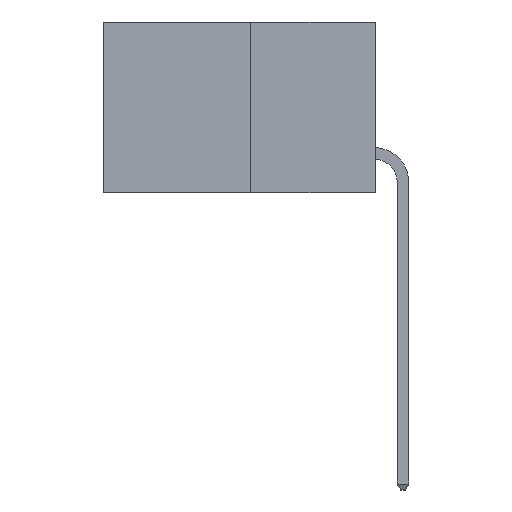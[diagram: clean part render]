
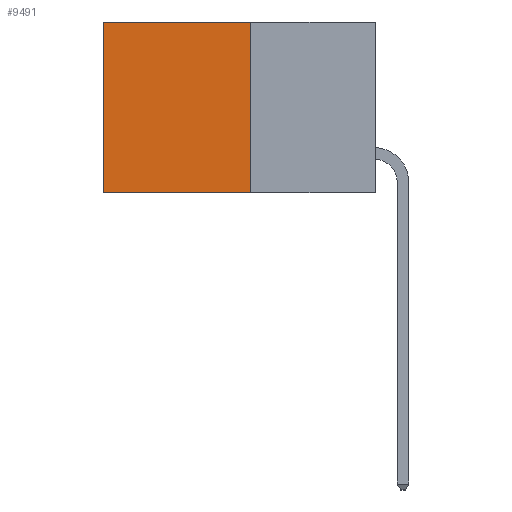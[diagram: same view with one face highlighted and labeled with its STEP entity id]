
A CAD part, left-side view. The second image highlights one B-rep face of the part: STEP entity #9491.
In plain terms, the highlighted planar face has unit normal (-1, 0, 0).
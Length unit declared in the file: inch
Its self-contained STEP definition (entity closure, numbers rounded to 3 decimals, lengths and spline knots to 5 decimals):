
#1117 = VECTOR ( 'NONE', #10026, 39.37008 ) ;
#1329 = VERTEX_POINT ( 'NONE', #5343 ) ;
#1611 = EDGE_CURVE ( 'NONE', #6706, #4238, #9862, .T. ) ;
#2186 = ORIENTED_EDGE ( 'NONE', *, *, #1611, .T. ) ;
#2219 = CARTESIAN_POINT ( 'NONE',  ( 0.277, 0.27, -0.37 ) ) ;
#2989 = VECTOR ( 'NONE', #11849, 39.37008 ) ;
#3197 = VERTEX_POINT ( 'NONE', #16836 ) ;
#3988 = EDGE_LOOP ( 'NONE', ( #2186, #4881, #17295, #4494 ) ) ;
#4238 = VERTEX_POINT ( 'NONE', #9027 ) ;
#4494 = ORIENTED_EDGE ( 'NONE', *, *, #9228, .T. ) ;
#4640 = CARTESIAN_POINT ( 'NONE',  ( 0.277, 0.59, -0.37 ) ) ;
#4686 = CARTESIAN_POINT ( 'NONE',  ( 0.277, 0.27, -0.37 ) ) ;
#4731 = CARTESIAN_POINT ( 'NONE',  ( 0.277, 0.27, 0. ) ) ;
#4881 = ORIENTED_EDGE ( 'NONE', *, *, #5100, .F. ) ;
#5100 = EDGE_CURVE ( 'NONE', #3197, #4238, #17859, .T. ) ;
#5343 = CARTESIAN_POINT ( 'NONE',  ( 0.277, 0.27, 0. ) ) ;
#5530 = VECTOR ( 'NONE', #7672, 39.37008 ) ;
#6706 = VERTEX_POINT ( 'NONE', #14539 ) ;
#6715 = DIRECTION ( 'NONE',  ( 0., 0., -1. ) ) ;
#6856 = AXIS2_PLACEMENT_3D ( 'NONE', #2219, #15010, #6715 ) ;
#7672 = DIRECTION ( 'NONE',  ( 0., 1., 0. ) ) ;
#9027 = CARTESIAN_POINT ( 'NONE',  ( 0.277, 0.59, -0.37 ) ) ;
#9123 = FACE_OUTER_BOUND ( 'NONE', #3988, .T. ) ;
#9228 = EDGE_CURVE ( 'NONE', #1329, #6706, #16568, .T. ) ;
#9491 = ADVANCED_FACE ( 'NONE', ( #9123 ), #9525, .F. ) ;
#9525 = PLANE ( 'NONE',  #6856 ) ;
#9862 = LINE ( 'NONE', #4640, #2989 ) ;
#10026 = DIRECTION ( 'NONE',  ( 0., 0., -1. ) ) ;
#11402 = CARTESIAN_POINT ( 'NONE',  ( 0.277, 0.27, -0.37 ) ) ;
#11849 = DIRECTION ( 'NONE',  ( 0., 0., -1. ) ) ;
#12623 = LINE ( 'NONE', #11402, #1117 ) ;
#14234 = VECTOR ( 'NONE', #16875, 39.37008 ) ;
#14539 = CARTESIAN_POINT ( 'NONE',  ( 0.277, 0.59, 0. ) ) ;
#15010 = DIRECTION ( 'NONE',  ( 1., 0., 0. ) ) ;
#15801 = EDGE_CURVE ( 'NONE', #1329, #3197, #12623, .T. ) ;
#16568 = LINE ( 'NONE', #4731, #5530 ) ;
#16836 = CARTESIAN_POINT ( 'NONE',  ( 0.277, 0.27, -0.37 ) ) ;
#16875 = DIRECTION ( 'NONE',  ( 0., 1., 0. ) ) ;
#17295 = ORIENTED_EDGE ( 'NONE', *, *, #15801, .F. ) ;
#17859 = LINE ( 'NONE', #4686, #14234 ) ;
